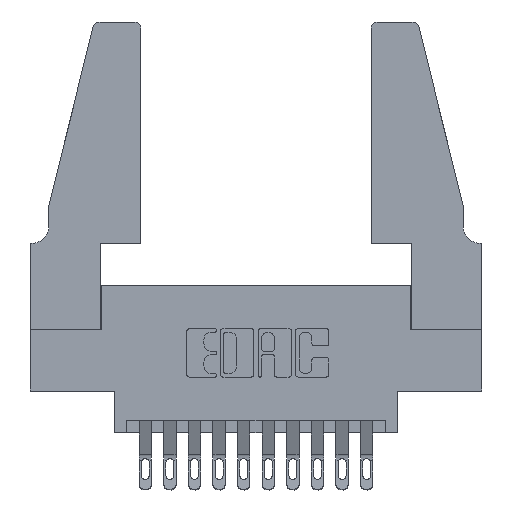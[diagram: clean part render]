
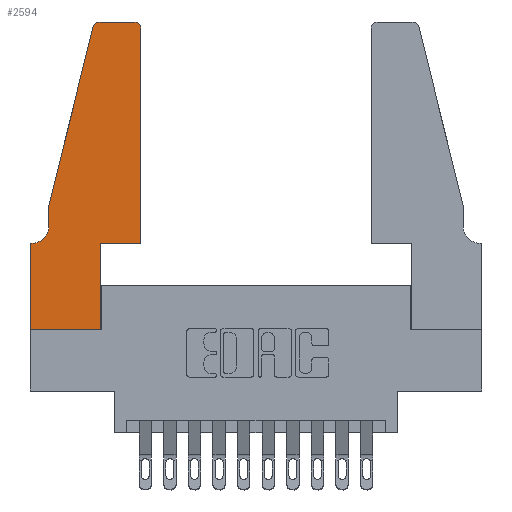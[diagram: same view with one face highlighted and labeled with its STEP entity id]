
A CAD part, top view. The second image highlights one B-rep face of the part: STEP entity #2594.
In plain terms, the highlighted planar face has unit normal (0, 0, 1).
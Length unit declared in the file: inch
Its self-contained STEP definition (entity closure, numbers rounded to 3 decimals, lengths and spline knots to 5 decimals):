
#59 = CARTESIAN_POINT ( 'NONE',  ( 0., 0., 0.37 ) ) ;
#146 = DIRECTION ( 'NONE',  ( 1., 0., 0. ) ) ;
#338 = VECTOR ( 'NONE', #146, 39.37008 ) ;
#369 = EDGE_CURVE ( 'NONE', #5234, #12861, #2530, .T. ) ;
#436 = VERTEX_POINT ( 'NONE', #7542 ) ;
#494 = DIRECTION ( 'NONE',  ( 1., 0., 0. ) ) ;
#641 = EDGE_CURVE ( 'NONE', #11541, #5234, #3772, .T. ) ;
#642 = DIRECTION ( 'NONE',  ( 0., 0., 1. ) ) ;
#653 = VECTOR ( 'NONE', #11400, 39.37008 ) ;
#668 = VERTEX_POINT ( 'NONE', #59 ) ;
#713 = ORIENTED_EDGE ( 'NONE', *, *, #13200, .T. ) ;
#715 = EDGE_CURVE ( 'NONE', #2838, #7608, #6997, .T. ) ;
#833 = VECTOR ( 'NONE', #13045, 39.37008 ) ;
#923 = VECTOR ( 'NONE', #6824, 39.37008 ) ;
#972 = CARTESIAN_POINT ( 'NONE',  ( 0.0055, 0.42, 0.37 ) ) ;
#994 = ORIENTED_EDGE ( 'NONE', *, *, #10271, .T. ) ;
#1546 = ORIENTED_EDGE ( 'NONE', *, *, #1703, .T. ) ;
#1703 = EDGE_CURVE ( 'NONE', #6532, #4361, #14766, .T. ) ;
#1963 = VECTOR ( 'NONE', #3648, 39.37008 ) ;
#2041 = CARTESIAN_POINT ( 'NONE',  ( 0., 0.35, 0.37 ) ) ;
#2381 = EDGE_CURVE ( 'NONE', #4361, #2838, #3720, .T. ) ;
#2530 = LINE ( 'NONE', #11861, #10876 ) ;
#2594 = ADVANCED_FACE ( 'NONE', ( #6881 ), #14556, .T. ) ;
#2723 = CARTESIAN_POINT ( 'NONE',  ( 0.0755, 0.5, 0.37 ) ) ;
#2838 = VERTEX_POINT ( 'NONE', #12973 ) ;
#3297 = ORIENTED_EDGE ( 'NONE', *, *, #13141, .T. ) ;
#3484 = CARTESIAN_POINT ( 'NONE',  ( 0.284, 1.25, 0.37 ) ) ;
#3648 = DIRECTION ( 'NONE',  ( -0.239, -0.971, 0. ) ) ;
#3704 = EDGE_CURVE ( 'NONE', #12861, #668, #4532, .T. ) ;
#3720 = CIRCLE ( 'NONE', #12297, 0.03 ) ;
#3772 = CIRCLE ( 'NONE', #12409, 0.07 ) ;
#3989 = LINE ( 'NONE', #13566, #12728 ) ;
#4115 = LINE ( 'NONE', #12789, #338 ) ;
#4195 = LINE ( 'NONE', #5257, #8124 ) ;
#4361 = VERTEX_POINT ( 'NONE', #3484 ) ;
#4532 = LINE ( 'NONE', #7918, #923 ) ;
#4753 = VERTEX_POINT ( 'NONE', #8988 ) ;
#4759 = CARTESIAN_POINT ( 'NONE',  ( 0.0755, 0.5, 0.37 ) ) ;
#4810 = CARTESIAN_POINT ( 'NONE',  ( 0.0755, 0.42, 0.37 ) ) ;
#5014 = EDGE_CURVE ( 'NONE', #668, #436, #4115, .T. ) ;
#5212 = ORIENTED_EDGE ( 'NONE', *, *, #641, .T. ) ;
#5234 = VERTEX_POINT ( 'NONE', #6320 ) ;
#5257 = CARTESIAN_POINT ( 'NONE',  ( 0.0755, 0.5, 0.37 ) ) ;
#5363 = ORIENTED_EDGE ( 'NONE', *, *, #369, .T. ) ;
#5514 = ORIENTED_EDGE ( 'NONE', *, *, #715, .T. ) ;
#5692 = DIRECTION ( 'NONE',  ( 0., 0., -1. ) ) ;
#6063 = CARTESIAN_POINT ( 'NONE',  ( 0., 0.35, 0.37 ) ) ;
#6113 = CARTESIAN_POINT ( 'NONE',  ( 0.2865, 0.35, 0.37 ) ) ;
#6118 = DIRECTION ( 'NONE',  ( 1., 0., 0. ) ) ;
#6320 = CARTESIAN_POINT ( 'NONE',  ( 0.0055, 0.35, 0.37 ) ) ;
#6326 = VECTOR ( 'NONE', #13434, 39.37008 ) ;
#6375 = EDGE_LOOP ( 'NONE', ( #1546, #8120, #5514, #12814, #5212, #5363, #12936, #8929, #3297, #994, #713, #8697 ) ) ;
#6532 = VERTEX_POINT ( 'NONE', #14095 ) ;
#6640 = CARTESIAN_POINT ( 'NONE',  ( 0.2865, 0.35, 0.37 ) ) ;
#6824 = DIRECTION ( 'NONE',  ( 0., -1., 0. ) ) ;
#6881 = FACE_OUTER_BOUND ( 'NONE', #6375, .T. ) ;
#6997 = LINE ( 'NONE', #4759, #1963 ) ;
#7434 = CARTESIAN_POINT ( 'NONE',  ( 0.4505, 0.35, 0.37 ) ) ;
#7528 = DIRECTION ( 'NONE',  ( 0., -1., 0. ) ) ;
#7542 = CARTESIAN_POINT ( 'NONE',  ( 0.2865, 0., 0.37 ) ) ;
#7608 = VERTEX_POINT ( 'NONE', #2723 ) ;
#7918 = CARTESIAN_POINT ( 'NONE',  ( 0., 0., 0.37 ) ) ;
#7930 = DIRECTION ( 'NONE',  ( 0., 1., 0. ) ) ;
#8120 = ORIENTED_EDGE ( 'NONE', *, *, #2381, .T. ) ;
#8124 = VECTOR ( 'NONE', #7528, 39.37008 ) ;
#8423 = VERTEX_POINT ( 'NONE', #14350 ) ;
#8471 = CIRCLE ( 'NONE', #12763, 0.03 ) ;
#8697 = ORIENTED_EDGE ( 'NONE', *, *, #8857, .T. ) ;
#8857 = EDGE_CURVE ( 'NONE', #8423, #6532, #8471, .T. ) ;
#8929 = ORIENTED_EDGE ( 'NONE', *, *, #5014, .T. ) ;
#8988 = CARTESIAN_POINT ( 'NONE',  ( 0.4505, 0.35, 0.37 ) ) ;
#10089 = DIRECTION ( 'NONE',  ( -1., 0., 0. ) ) ;
#10248 = CARTESIAN_POINT ( 'NONE',  ( 0.2605, 1.25, 0.37 ) ) ;
#10271 = EDGE_CURVE ( 'NONE', #10481, #4753, #10467, .T. ) ;
#10376 = LINE ( 'NONE', #6640, #6326 ) ;
#10467 = LINE ( 'NONE', #7434, #833 ) ;
#10481 = VERTEX_POINT ( 'NONE', #6113 ) ;
#10718 = CARTESIAN_POINT ( 'NONE',  ( 0.4205, 1.22, 0.37 ) ) ;
#10876 = VECTOR ( 'NONE', #12821, 39.37008 ) ;
#11400 = DIRECTION ( 'NONE',  ( -1., 0., 0. ) ) ;
#11541 = VERTEX_POINT ( 'NONE', #4810 ) ;
#11624 = DIRECTION ( 'NONE',  ( 0., 0., 1. ) ) ;
#11847 = EDGE_CURVE ( 'NONE', #7608, #11541, #4195, .T. ) ;
#11861 = CARTESIAN_POINT ( 'NONE',  ( 0.0755, 0.35, 0.37 ) ) ;
#12297 = AXIS2_PLACEMENT_3D ( 'NONE', #13033, #14158, #494 ) ;
#12409 = AXIS2_PLACEMENT_3D ( 'NONE', #972, #5692, #10089 ) ;
#12728 = VECTOR ( 'NONE', #7930, 39.37008 ) ;
#12763 = AXIS2_PLACEMENT_3D ( 'NONE', #10718, #642, #13044 ) ;
#12789 = CARTESIAN_POINT ( 'NONE',  ( 0., 0., 0.37 ) ) ;
#12814 = ORIENTED_EDGE ( 'NONE', *, *, #11847, .T. ) ;
#12821 = DIRECTION ( 'NONE',  ( -1., 0., 0. ) ) ;
#12861 = VERTEX_POINT ( 'NONE', #6063 ) ;
#12936 = ORIENTED_EDGE ( 'NONE', *, *, #3704, .T. ) ;
#12973 = CARTESIAN_POINT ( 'NONE',  ( 0.25487, 1.22718, 0.37 ) ) ;
#13033 = CARTESIAN_POINT ( 'NONE',  ( 0.284, 1.22, 0.37 ) ) ;
#13044 = DIRECTION ( 'NONE',  ( 1., 0., 0. ) ) ;
#13045 = DIRECTION ( 'NONE',  ( 1., 0., 0. ) ) ;
#13141 = EDGE_CURVE ( 'NONE', #436, #10481, #10376, .T. ) ;
#13200 = EDGE_CURVE ( 'NONE', #4753, #8423, #3989, .T. ) ;
#13238 = AXIS2_PLACEMENT_3D ( 'NONE', #2041, #11624, #6118 ) ;
#13434 = DIRECTION ( 'NONE',  ( 0., 1., 0. ) ) ;
#13566 = CARTESIAN_POINT ( 'NONE',  ( 0.4505, 0.35, 0.37 ) ) ;
#14095 = CARTESIAN_POINT ( 'NONE',  ( 0.4205, 1.25, 0.37 ) ) ;
#14158 = DIRECTION ( 'NONE',  ( 0., 0., 1. ) ) ;
#14350 = CARTESIAN_POINT ( 'NONE',  ( 0.4505, 1.22, 0.37 ) ) ;
#14556 = PLANE ( 'NONE',  #13238 ) ;
#14766 = LINE ( 'NONE', #10248, #653 ) ;
